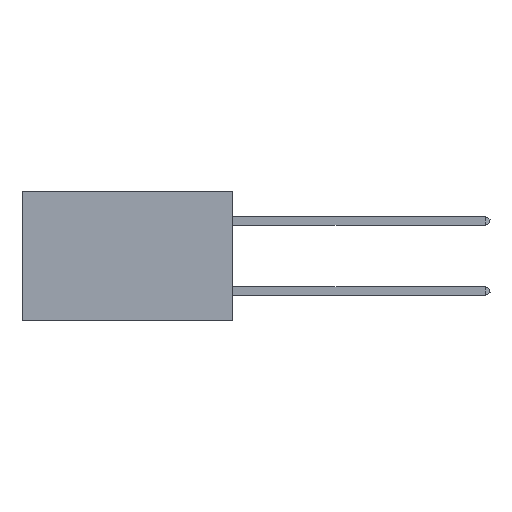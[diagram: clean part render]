
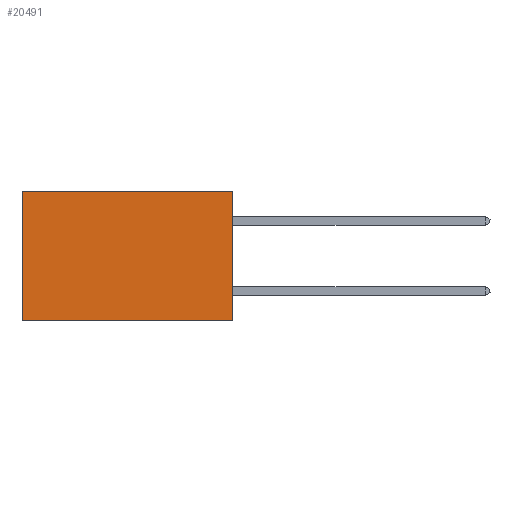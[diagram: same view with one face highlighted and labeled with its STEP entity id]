
A CAD part, left-side view. The second image highlights one B-rep face of the part: STEP entity #20491.
In plain terms, the highlighted planar face has unit normal (-1, 0, 0).
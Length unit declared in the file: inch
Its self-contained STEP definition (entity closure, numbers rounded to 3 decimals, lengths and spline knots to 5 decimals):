
#666 = CARTESIAN_POINT ( 'NONE',  ( 0.2875, 0.6, -0.37 ) ) ;
#1485 = EDGE_LOOP ( 'NONE', ( #30267, #1861, #19629, #15164 ) ) ;
#1861 = ORIENTED_EDGE ( 'NONE', *, *, #15276, .F. ) ;
#3481 = AXIS2_PLACEMENT_3D ( 'NONE', #21529, #21254, #6534 ) ;
#5018 = VERTEX_POINT ( 'NONE', #15237 ) ;
#6534 = DIRECTION ( 'NONE',  ( 0., 0., -1. ) ) ;
#7069 = EDGE_CURVE ( 'NONE', #5018, #17214, #18451, .T. ) ;
#7451 = DIRECTION ( 'NONE',  ( 0., 1., 0. ) ) ;
#8749 = LINE ( 'NONE', #29611, #12713 ) ;
#9478 = LINE ( 'NONE', #28439, #27136 ) ;
#9690 = EDGE_CURVE ( 'NONE', #17214, #28909, #9478, .T. ) ;
#10575 = DIRECTION ( 'NONE',  ( 0., 0., -1. ) ) ;
#12713 = VECTOR ( 'NONE', #10575, 39.37008 ) ;
#12785 = CARTESIAN_POINT ( 'NONE',  ( 0.2875, 0., 0. ) ) ;
#14276 = VERTEX_POINT ( 'NONE', #29102 ) ;
#15164 = ORIENTED_EDGE ( 'NONE', *, *, #7069, .T. ) ;
#15237 = CARTESIAN_POINT ( 'NONE',  ( 0.2875, 0., 0. ) ) ;
#15276 = EDGE_CURVE ( 'NONE', #14276, #28909, #16268, .T. ) ;
#16268 = LINE ( 'NONE', #28900, #23717 ) ;
#17214 = VERTEX_POINT ( 'NONE', #30555 ) ;
#18451 = LINE ( 'NONE', #12785, #23287 ) ;
#19629 = ORIENTED_EDGE ( 'NONE', *, *, #21053, .F. ) ;
#20491 = ADVANCED_FACE ( 'NONE', ( #20522 ), #23455, .F. ) ;
#20522 = FACE_OUTER_BOUND ( 'NONE', #1485, .T. ) ;
#21053 = EDGE_CURVE ( 'NONE', #5018, #14276, #8749, .T. ) ;
#21254 = DIRECTION ( 'NONE',  ( 1., 0., 0. ) ) ;
#21529 = CARTESIAN_POINT ( 'NONE',  ( 0.2875, 0., 0. ) ) ;
#21530 = DIRECTION ( 'NONE',  ( 0., 0., -1. ) ) ;
#23287 = VECTOR ( 'NONE', #26745, 39.37008 ) ;
#23455 = PLANE ( 'NONE',  #3481 ) ;
#23717 = VECTOR ( 'NONE', #7451, 39.37008 ) ;
#26745 = DIRECTION ( 'NONE',  ( 0., 1., 0. ) ) ;
#27136 = VECTOR ( 'NONE', #21530, 39.37008 ) ;
#28439 = CARTESIAN_POINT ( 'NONE',  ( 0.2875, 0.6, 0. ) ) ;
#28900 = CARTESIAN_POINT ( 'NONE',  ( 0.2875, 0., -0.37 ) ) ;
#28909 = VERTEX_POINT ( 'NONE', #666 ) ;
#29102 = CARTESIAN_POINT ( 'NONE',  ( 0.2875, 0., -0.37 ) ) ;
#29611 = CARTESIAN_POINT ( 'NONE',  ( 0.2875, 0., 0. ) ) ;
#30267 = ORIENTED_EDGE ( 'NONE', *, *, #9690, .T. ) ;
#30555 = CARTESIAN_POINT ( 'NONE',  ( 0.2875, 0.6, 0. ) ) ;
